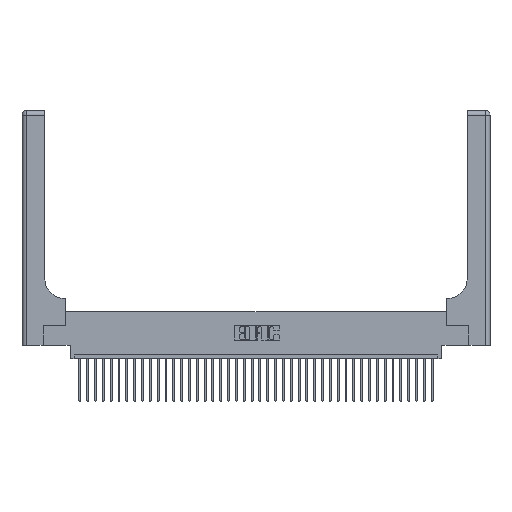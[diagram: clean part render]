
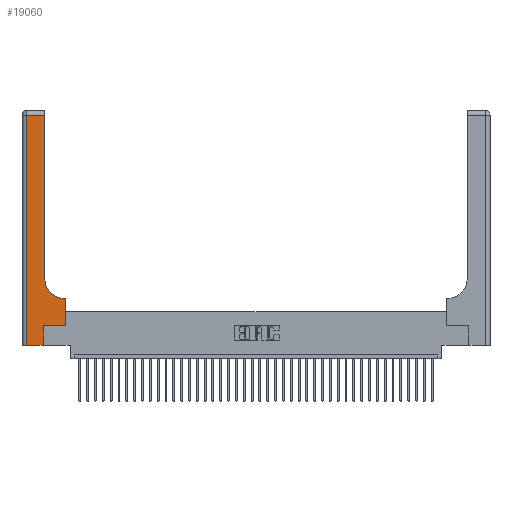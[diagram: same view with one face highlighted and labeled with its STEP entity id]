
A CAD part, top view. The second image highlights one B-rep face of the part: STEP entity #19060.
In plain terms, the highlighted planar face has unit normal (0, 0, 1).
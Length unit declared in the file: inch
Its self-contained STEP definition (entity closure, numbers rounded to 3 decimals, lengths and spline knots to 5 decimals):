
#236 = CARTESIAN_POINT ( 'NONE',  ( 0.2915, 2.94, 0.37 ) ) ;
#408 = LINE ( 'NONE', #25731, #24228 ) ;
#1400 = DIRECTION ( 'NONE',  ( -1., 0., 0. ) ) ;
#1735 = DIRECTION ( 'NONE',  ( 0., 0., -1. ) ) ;
#2437 = CARTESIAN_POINT ( 'NONE',  ( 0.269, 0., 0.37 ) ) ;
#2792 = ORIENTED_EDGE ( 'NONE', *, *, #34817, .T. ) ;
#2948 = CARTESIAN_POINT ( 'NONE',  ( 0.269, 0.25, 0.37 ) ) ;
#3645 = VERTEX_POINT ( 'NONE', #22310 ) ;
#3754 = DIRECTION ( 'NONE',  ( 0., 1., 0. ) ) ;
#4772 = CARTESIAN_POINT ( 'NONE',  ( 0., 3., 0.37 ) ) ;
#5545 = CARTESIAN_POINT ( 'NONE',  ( 0.06, 3., 0.37 ) ) ;
#6776 = ORIENTED_EDGE ( 'NONE', *, *, #19641, .T. ) ;
#6845 = ORIENTED_EDGE ( 'NONE', *, *, #8878, .T. ) ;
#7420 = VERTEX_POINT ( 'NONE', #38511 ) ;
#7685 = EDGE_CURVE ( 'NONE', #21388, #22442, #15580, .T. ) ;
#7886 = ORIENTED_EDGE ( 'NONE', *, *, #7685, .T. ) ;
#7989 = CARTESIAN_POINT ( 'NONE',  ( 0., 0., 0.37 ) ) ;
#8878 = EDGE_CURVE ( 'NONE', #22442, #11551, #25484, .T. ) ;
#9134 = LINE ( 'NONE', #7989, #24801 ) ;
#9396 = EDGE_CURVE ( 'NONE', #30441, #7420, #18822, .T. ) ;
#9562 = ORIENTED_EDGE ( 'NONE', *, *, #31539, .T. ) ;
#11152 = LINE ( 'NONE', #37226, #17346 ) ;
#11551 = VERTEX_POINT ( 'NONE', #28439 ) ;
#11617 = VERTEX_POINT ( 'NONE', #16552 ) ;
#12432 = VECTOR ( 'NONE', #26960, 39.37008 ) ;
#12580 = VECTOR ( 'NONE', #13049, 39.37008 ) ;
#12619 = DIRECTION ( 'NONE',  ( -1., 0., 0. ) ) ;
#12895 = LINE ( 'NONE', #5545, #12432 ) ;
#12913 = DIRECTION ( 'NONE',  ( 0., 1., 0. ) ) ;
#13049 = DIRECTION ( 'NONE',  ( 1., 0., 0. ) ) ;
#13172 = CARTESIAN_POINT ( 'NONE',  ( 0.269, 0., 0.37 ) ) ;
#13423 = FACE_OUTER_BOUND ( 'NONE', #22366, .T. ) ;
#13532 = DIRECTION ( 'NONE',  ( -1., 0., 0. ) ) ;
#15269 = EDGE_CURVE ( 'NONE', #7420, #30917, #36354, .T. ) ;
#15508 = AXIS2_PLACEMENT_3D ( 'NONE', #25433, #22798, #22029 ) ;
#15580 = LINE ( 'NONE', #13172, #30812 ) ;
#16552 = CARTESIAN_POINT ( 'NONE',  ( 0.06, 0., 0.37 ) ) ;
#16637 = DIRECTION ( 'NONE',  ( 1., 0., 0. ) ) ;
#16647 = EDGE_CURVE ( 'NONE', #11617, #21388, #9134, .T. ) ;
#16776 = ORIENTED_EDGE ( 'NONE', *, *, #16647, .T. ) ;
#17346 = VECTOR ( 'NONE', #12619, 39.37008 ) ;
#17492 = ORIENTED_EDGE ( 'NONE', *, *, #15269, .T. ) ;
#18822 = CIRCLE ( 'NONE', #15508, 0.25 ) ;
#19060 = ADVANCED_FACE ( 'NONE', ( #13423 ), #19836, .F. ) ;
#19641 = EDGE_CURVE ( 'NONE', #3645, #11617, #12895, .T. ) ;
#19836 = PLANE ( 'NONE',  #24292 ) ;
#20374 = DIRECTION ( 'NONE',  ( 0., 1., 0. ) ) ;
#20639 = CARTESIAN_POINT ( 'NONE',  ( 0.5585, 0.25, 0.37 ) ) ;
#21084 = VERTEX_POINT ( 'NONE', #33270 ) ;
#21388 = VERTEX_POINT ( 'NONE', #2437 ) ;
#22029 = DIRECTION ( 'NONE',  ( 1., 0., 0. ) ) ;
#22310 = CARTESIAN_POINT ( 'NONE',  ( 0.06, 2.94, 0.37 ) ) ;
#22366 = EDGE_LOOP ( 'NONE', ( #17492, #2792, #6776, #16776, #7886, #6845, #27311, #9562, #32963 ) ) ;
#22442 = VERTEX_POINT ( 'NONE', #2948 ) ;
#22798 = DIRECTION ( 'NONE',  ( 0., 0., -1. ) ) ;
#24228 = VECTOR ( 'NONE', #1400, 39.37008 ) ;
#24292 = AXIS2_PLACEMENT_3D ( 'NONE', #4772, #1735, #13532 ) ;
#24801 = VECTOR ( 'NONE', #16637, 39.37008 ) ;
#25185 = EDGE_CURVE ( 'NONE', #11551, #21084, #27863, .T. ) ;
#25433 = CARTESIAN_POINT ( 'NONE',  ( 0.5415, 0.85, 0.37 ) ) ;
#25484 = LINE ( 'NONE', #27850, #12580 ) ;
#25731 = CARTESIAN_POINT ( 'NONE',  ( 0., 2.94, 0.37 ) ) ;
#26955 = VECTOR ( 'NONE', #20374, 39.37008 ) ;
#26960 = DIRECTION ( 'NONE',  ( 0., -1., 0. ) ) ;
#27311 = ORIENTED_EDGE ( 'NONE', *, *, #25185, .T. ) ;
#27849 = CARTESIAN_POINT ( 'NONE',  ( 0.2915, 3., 0.37 ) ) ;
#27850 = CARTESIAN_POINT ( 'NONE',  ( 0.269, 0.25, 0.37 ) ) ;
#27863 = LINE ( 'NONE', #20639, #26955 ) ;
#28439 = CARTESIAN_POINT ( 'NONE',  ( 0.5585, 0.25, 0.37 ) ) ;
#30441 = VERTEX_POINT ( 'NONE', #33308 ) ;
#30812 = VECTOR ( 'NONE', #3754, 39.37008 ) ;
#30917 = VERTEX_POINT ( 'NONE', #236 ) ;
#31539 = EDGE_CURVE ( 'NONE', #21084, #30441, #11152, .T. ) ;
#32963 = ORIENTED_EDGE ( 'NONE', *, *, #9396, .T. ) ;
#33270 = CARTESIAN_POINT ( 'NONE',  ( 0.5585, 0.6, 0.37 ) ) ;
#33308 = CARTESIAN_POINT ( 'NONE',  ( 0.5415, 0.6, 0.37 ) ) ;
#34817 = EDGE_CURVE ( 'NONE', #30917, #3645, #408, .T. ) ;
#35920 = VECTOR ( 'NONE', #12913, 39.37008 ) ;
#36354 = LINE ( 'NONE', #27849, #35920 ) ;
#37226 = CARTESIAN_POINT ( 'NONE',  ( 0.2915, 0.6, 0.37 ) ) ;
#38511 = CARTESIAN_POINT ( 'NONE',  ( 0.2915, 0.85, 0.37 ) ) ;
